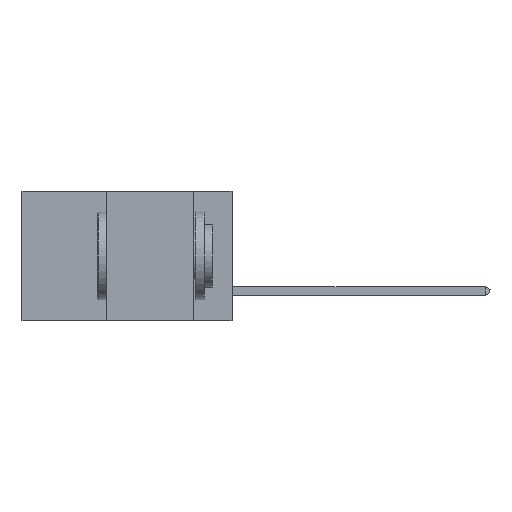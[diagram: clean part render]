
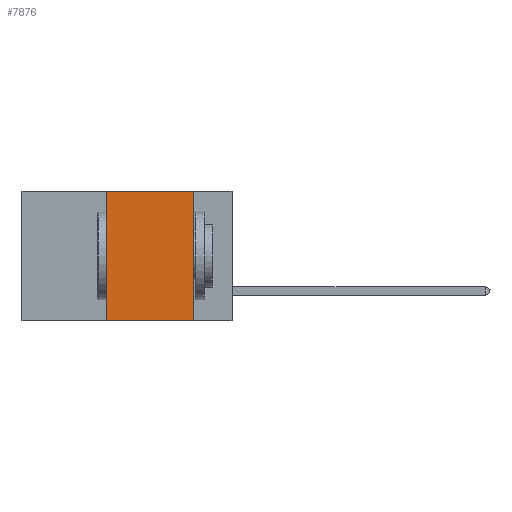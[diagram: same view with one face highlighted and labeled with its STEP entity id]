
A CAD part, left-side view. The second image highlights one B-rep face of the part: STEP entity #7876.
In plain terms, the highlighted planar face has unit normal (-1, 0, 0).
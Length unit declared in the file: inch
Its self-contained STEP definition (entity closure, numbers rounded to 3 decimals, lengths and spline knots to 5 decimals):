
#67 = DIRECTION ( 'NONE',  ( 0., 0., 1. ) ) ;
#219 = CARTESIAN_POINT ( 'NONE',  ( 0., 0.6, 0. ) ) ;
#1009 = LINE ( 'NONE', #3660, #4893 ) ;
#1065 = VECTOR ( 'NONE', #67, 39.37008 ) ;
#1101 = DIRECTION ( 'NONE',  ( 1., 0., 0. ) ) ;
#1239 = EDGE_CURVE ( 'NONE', #5877, #6354, #11782, .T. ) ;
#1845 = FACE_OUTER_BOUND ( 'NONE', #8533, .T. ) ;
#2035 = DIRECTION ( 'NONE',  ( 0., -1., 0. ) ) ;
#2234 = LINE ( 'NONE', #10061, #1065 ) ;
#2751 = CARTESIAN_POINT ( 'NONE',  ( 0., 0.11, 0. ) ) ;
#3660 = CARTESIAN_POINT ( 'NONE',  ( 0., 0.6, -0.37 ) ) ;
#3905 = VERTEX_POINT ( 'NONE', #9255 ) ;
#4004 = CARTESIAN_POINT ( 'NONE',  ( 0., 0.11, -0.37 ) ) ;
#4634 = VECTOR ( 'NONE', #11106, 39.37008 ) ;
#4849 = ORIENTED_EDGE ( 'NONE', *, *, #8886, .F. ) ;
#4893 = VECTOR ( 'NONE', #7410, 39.37008 ) ;
#5383 = VECTOR ( 'NONE', #2035, 39.37008 ) ;
#5398 = CARTESIAN_POINT ( 'NONE',  ( 0., 0.11, 0. ) ) ;
#5877 = VERTEX_POINT ( 'NONE', #10823 ) ;
#5925 = ORIENTED_EDGE ( 'NONE', *, *, #11385, .T. ) ;
#6354 = VERTEX_POINT ( 'NONE', #5398 ) ;
#6470 = LINE ( 'NONE', #2751, #4634 ) ;
#7410 = DIRECTION ( 'NONE',  ( 0., -1., 0. ) ) ;
#7478 = DIRECTION ( 'NONE',  ( 0., 0., -1. ) ) ;
#7876 = ADVANCED_FACE ( 'NONE', ( #1845 ), #11249, .F. ) ;
#8301 = AXIS2_PLACEMENT_3D ( 'NONE', #219, #1101, #7478 ) ;
#8378 = ORIENTED_EDGE ( 'NONE', *, *, #1239, .F. ) ;
#8530 = ORIENTED_EDGE ( 'NONE', *, *, #10073, .F. ) ;
#8533 = EDGE_LOOP ( 'NONE', ( #8530, #8378, #4849, #5925 ) ) ;
#8886 = EDGE_CURVE ( 'NONE', #3905, #5877, #2234, .T. ) ;
#9255 = CARTESIAN_POINT ( 'NONE',  ( 0., 0.36, -0.37 ) ) ;
#9389 = CARTESIAN_POINT ( 'NONE',  ( 0., 0.6, 0. ) ) ;
#10061 = CARTESIAN_POINT ( 'NONE',  ( 0., 0.36, 0. ) ) ;
#10073 = EDGE_CURVE ( 'NONE', #6354, #10576, #6470, .T. ) ;
#10576 = VERTEX_POINT ( 'NONE', #4004 ) ;
#10823 = CARTESIAN_POINT ( 'NONE',  ( 0., 0.36, 0. ) ) ;
#11106 = DIRECTION ( 'NONE',  ( 0., 0., -1. ) ) ;
#11249 = PLANE ( 'NONE',  #8301 ) ;
#11385 = EDGE_CURVE ( 'NONE', #3905, #10576, #1009, .T. ) ;
#11782 = LINE ( 'NONE', #9389, #5383 ) ;
